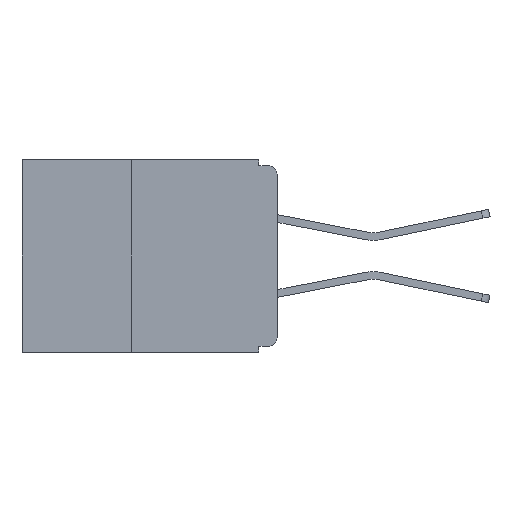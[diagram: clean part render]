
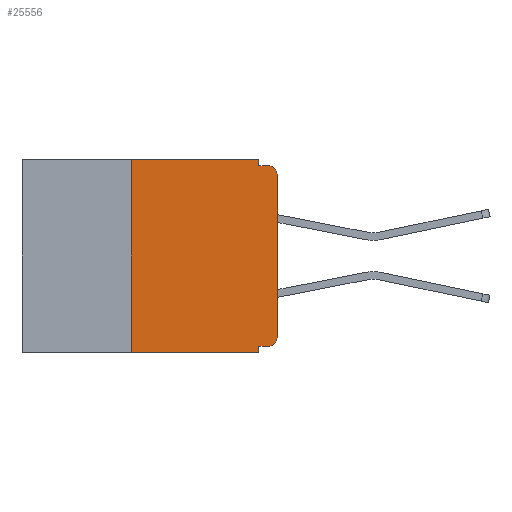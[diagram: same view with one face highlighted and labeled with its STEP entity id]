
A CAD part, left-side view. The second image highlights one B-rep face of the part: STEP entity #25556.
In plain terms, the highlighted planar face has unit normal (-1, 0, 0).
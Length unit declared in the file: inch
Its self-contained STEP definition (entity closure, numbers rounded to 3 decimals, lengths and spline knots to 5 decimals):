
#375 = EDGE_CURVE ( 'NONE', #14913, #21384, #13559, .T. ) ;
#411 = VERTEX_POINT ( 'NONE', #27538 ) ;
#631 = EDGE_CURVE ( 'NONE', #12578, #26311, #13880, .T. ) ;
#869 = CARTESIAN_POINT ( 'NONE',  ( 0., 0.031, -0.33 ) ) ;
#1134 = AXIS2_PLACEMENT_3D ( 'NONE', #12987, #27064, #15152 ) ;
#1634 = VECTOR ( 'NONE', #10310, 39.37008 ) ;
#1718 = VECTOR ( 'NONE', #17055, 39.37008 ) ;
#2023 = PLANE ( 'NONE',  #13353 ) ;
#2226 = ORIENTED_EDGE ( 'NONE', *, *, #16538, .T. ) ;
#2583 = ORIENTED_EDGE ( 'NONE', *, *, #16745, .T. ) ;
#3379 = VERTEX_POINT ( 'NONE', #869 ) ;
#3916 = VECTOR ( 'NONE', #7605, 39.37008 ) ;
#3964 = CARTESIAN_POINT ( 'NONE',  ( 0., 0.015, -0.01 ) ) ;
#5388 = CARTESIAN_POINT ( 'NONE',  ( 0., 0.031, 0. ) ) ;
#5610 = FACE_OUTER_BOUND ( 'NONE', #16789, .T. ) ;
#6366 = DIRECTION ( 'NONE',  ( 1., 0., 0. ) ) ;
#6713 = CARTESIAN_POINT ( 'NONE',  ( 0., 0.25, -0.33 ) ) ;
#6720 = ORIENTED_EDGE ( 'NONE', *, *, #19270, .T. ) ;
#7325 = CARTESIAN_POINT ( 'NONE',  ( 0., 0., -0.32 ) ) ;
#7605 = DIRECTION ( 'NONE',  ( 0., 0., -1. ) ) ;
#7632 = CARTESIAN_POINT ( 'NONE',  ( 0., 0.031, -0.33 ) ) ;
#7771 = ORIENTED_EDGE ( 'NONE', *, *, #12416, .F. ) ;
#8299 = VERTEX_POINT ( 'NONE', #11854 ) ;
#8779 = LINE ( 'NONE', #9343, #19440 ) ;
#8869 = DIRECTION ( 'NONE',  ( 0., 0., 1. ) ) ;
#8993 = CARTESIAN_POINT ( 'NONE',  ( 0., 0., -0.01 ) ) ;
#9343 = CARTESIAN_POINT ( 'NONE',  ( 0., 0.437, -0.33 ) ) ;
#9408 = ORIENTED_EDGE ( 'NONE', *, *, #9576, .F. ) ;
#9576 = EDGE_CURVE ( 'NONE', #26311, #27092, #20991, .T. ) ;
#9591 = LINE ( 'NONE', #6713, #20207 ) ;
#9765 = ORIENTED_EDGE ( 'NONE', *, *, #17905, .F. ) ;
#10310 = DIRECTION ( 'NONE',  ( 0., -1., 0. ) ) ;
#10359 = VECTOR ( 'NONE', #20049, 39.37008 ) ;
#11047 = VERTEX_POINT ( 'NONE', #3964 ) ;
#11854 = CARTESIAN_POINT ( 'NONE',  ( 0., 0.25, -0.33 ) ) ;
#12416 = EDGE_CURVE ( 'NONE', #8299, #12578, #9591, .T. ) ;
#12578 = VERTEX_POINT ( 'NONE', #17821 ) ;
#12738 = CARTESIAN_POINT ( 'NONE',  ( 0., 0., 0. ) ) ;
#12987 = CARTESIAN_POINT ( 'NONE',  ( 0., 0.015, -0.025 ) ) ;
#13154 = VERTEX_POINT ( 'NONE', #26262 ) ;
#13353 = AXIS2_PLACEMENT_3D ( 'NONE', #27555, #6366, #17134 ) ;
#13449 = CARTESIAN_POINT ( 'NONE',  ( 0., 0.031, 0. ) ) ;
#13559 = CIRCLE ( 'NONE', #17540, 0.015 ) ;
#13844 = CARTESIAN_POINT ( 'NONE',  ( 0., 0.015, -0.305 ) ) ;
#13880 = LINE ( 'NONE', #26788, #1634 ) ;
#13965 = LINE ( 'NONE', #12738, #1718 ) ;
#14913 = VERTEX_POINT ( 'NONE', #24005 ) ;
#15152 = DIRECTION ( 'NONE',  ( 0., 0., -1. ) ) ;
#15268 = DIRECTION ( 'NONE',  ( -1., 0., 0. ) ) ;
#16538 = EDGE_CURVE ( 'NONE', #411, #11047, #19112, .T. ) ;
#16609 = LINE ( 'NONE', #7632, #27076 ) ;
#16745 = EDGE_CURVE ( 'NONE', #8299, #3379, #8779, .T. ) ;
#16789 = EDGE_LOOP ( 'NONE', ( #6720, #2226, #20035, #9408, #26932, #7771, #2583, #19729, #9765, #26624 ) ) ;
#17055 = DIRECTION ( 'NONE',  ( 0., 0., 1. ) ) ;
#17134 = DIRECTION ( 'NONE',  ( 0., 0., -1. ) ) ;
#17502 = DIRECTION ( 'NONE',  ( 0., -1., 0. ) ) ;
#17540 = AXIS2_PLACEMENT_3D ( 'NONE', #13844, #15268, #24459 ) ;
#17821 = CARTESIAN_POINT ( 'NONE',  ( 0., 0.25, 0. ) ) ;
#17905 = EDGE_CURVE ( 'NONE', #14913, #13154, #26551, .T. ) ;
#19112 = CIRCLE ( 'NONE', #1134, 0.015 ) ;
#19270 = EDGE_CURVE ( 'NONE', #21384, #411, #13965, .T. ) ;
#19331 = VECTOR ( 'NONE', #17502, 39.37008 ) ;
#19440 = VECTOR ( 'NONE', #19927, 39.37008 ) ;
#19729 = ORIENTED_EDGE ( 'NONE', *, *, #20936, .F. ) ;
#19927 = DIRECTION ( 'NONE',  ( 0., -1., 0. ) ) ;
#19968 = LINE ( 'NONE', #8993, #19331 ) ;
#20035 = ORIENTED_EDGE ( 'NONE', *, *, #25649, .F. ) ;
#20049 = DIRECTION ( 'NONE',  ( 0., 1., 0. ) ) ;
#20207 = VECTOR ( 'NONE', #8869, 39.37008 ) ;
#20936 = EDGE_CURVE ( 'NONE', #13154, #3379, #16609, .T. ) ;
#20991 = LINE ( 'NONE', #5388, #3916 ) ;
#21384 = VERTEX_POINT ( 'NONE', #26540 ) ;
#24005 = CARTESIAN_POINT ( 'NONE',  ( 0., 0.015, -0.32 ) ) ;
#24459 = DIRECTION ( 'NONE',  ( 0., 0., -1. ) ) ;
#24585 = DIRECTION ( 'NONE',  ( 0., 0., -1. ) ) ;
#24694 = CARTESIAN_POINT ( 'NONE',  ( 0., 0.031, -0.01 ) ) ;
#25556 = ADVANCED_FACE ( 'NONE', ( #5610 ), #2023, .F. ) ;
#25649 = EDGE_CURVE ( 'NONE', #27092, #11047, #19968, .T. ) ;
#26262 = CARTESIAN_POINT ( 'NONE',  ( 0., 0.031, -0.32 ) ) ;
#26311 = VERTEX_POINT ( 'NONE', #13449 ) ;
#26540 = CARTESIAN_POINT ( 'NONE',  ( 0., 0., -0.305 ) ) ;
#26551 = LINE ( 'NONE', #7325, #10359 ) ;
#26624 = ORIENTED_EDGE ( 'NONE', *, *, #375, .T. ) ;
#26788 = CARTESIAN_POINT ( 'NONE',  ( 0., 0.437, 0. ) ) ;
#26932 = ORIENTED_EDGE ( 'NONE', *, *, #631, .F. ) ;
#27064 = DIRECTION ( 'NONE',  ( -1., 0., 0. ) ) ;
#27076 = VECTOR ( 'NONE', #24585, 39.37008 ) ;
#27092 = VERTEX_POINT ( 'NONE', #24694 ) ;
#27538 = CARTESIAN_POINT ( 'NONE',  ( 0., 0., -0.025 ) ) ;
#27555 = CARTESIAN_POINT ( 'NONE',  ( 0., 0.437, 0. ) ) ;
